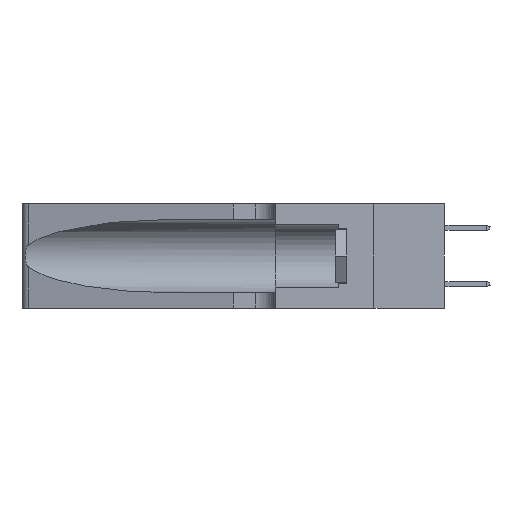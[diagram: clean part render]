
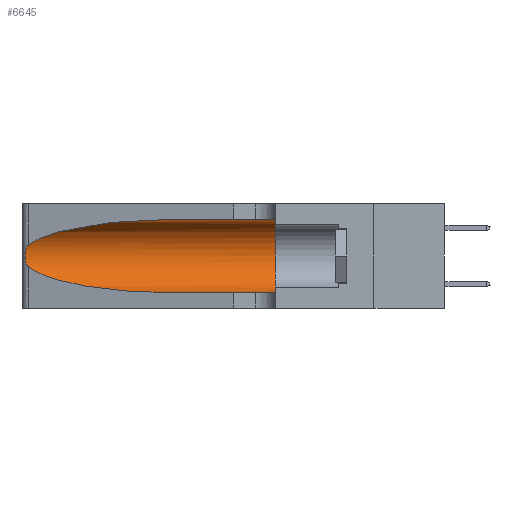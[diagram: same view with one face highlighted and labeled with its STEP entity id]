
A CAD part, left-side view. The second image highlights one B-rep face of the part: STEP entity #6645.
In plain terms, the highlighted cylindrical face has radius 3.308 mm (diameter 6.617 mm), a partial arc.
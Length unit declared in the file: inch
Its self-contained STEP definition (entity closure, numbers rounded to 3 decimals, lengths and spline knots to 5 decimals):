
#826 = VERTEX_POINT ( 'NONE', #35595 ) ;
#1830 = VECTOR ( 'NONE', #15714, 39.37008 ) ;
#2321 = DIRECTION ( 'NONE',  ( 0., -1., 0. ) ) ;
#2409 = ORIENTED_EDGE ( 'NONE', *, *, #2762, .T. ) ;
#2723 = CARTESIAN_POINT ( 'NONE',  ( 0.25487, 1.22718, 0.22369 ) ) ;
#2762 = EDGE_CURVE ( 'NONE', #18051, #28394, #26900, .T. ) ;
#2826 = EDGE_CURVE ( 'NONE', #33455, #10412, #31669, .T. ) ;
#3676 = CARTESIAN_POINT ( 'NONE',  ( 0.1305, 0.35, 0.185 ) ) ;
#4172 = CARTESIAN_POINT ( 'NONE',  ( 0.25555, 1.22994, 0.2215 ) ) ;
#4264 = B_SPLINE_CURVE_WITH_KNOTS ( 'NONE', 3,
 ( #15317, #4172, #23438, #17858, #7052, #34522, #20739, #18093, #4287, #26264, #34765, #12636, #17735, #20980 ),
 .UNSPECIFIED., .F., .F.,
 ( 4, 2, 2, 2, 2, 2, 4 ),
 ( 0., 0.00027, 0.00053, 0.00107, 0.0016, 0.00187, 0.00214 ),
 .UNSPECIFIED. ) ;
#4287 = CARTESIAN_POINT ( 'NONE',  ( 0.26017, 1.23833, 0.17102 ) ) ;
#4619 = EDGE_CURVE ( 'NONE', #826, #31121, #4264, .T. ) ;
#4683 = ORIENTED_EDGE ( 'NONE', *, *, #34054, .F. ) ;
#5385 = CARTESIAN_POINT ( 'NONE',  ( 0.1305, 0.72297, 0.31525 ) ) ;
#6645 = ADVANCED_FACE ( 'NONE', ( #24029 ), #17532, .F. ) ;
#7052 = CARTESIAN_POINT ( 'NONE',  ( 0.25854, 1.2359, 0.20912 ) ) ;
#8241 = CARTESIAN_POINT ( 'NONE',  ( 0.25487, 1.22718, 0.14631 ) ) ;
#9225 = ORIENTED_EDGE ( 'NONE', *, *, #15593, .T. ) ;
#9438 = AXIS2_PLACEMENT_3D ( 'NONE', #3676, #31109, #22939 ) ;
#10412 = VERTEX_POINT ( 'NONE', #28890 ) ;
#12636 = CARTESIAN_POINT ( 'NONE',  ( 0.25639, 1.23186, 0.15144 ) ) ;
#13640 = CARTESIAN_POINT ( 'NONE',  ( 0.18966, 0.96281, 0.31525 ) ) ;
#13798 = ORIENTED_EDGE ( 'NONE', *, *, #30500, .T. ) ;
#14192 = CARTESIAN_POINT ( 'NONE',  ( 0.1305, 0.35, 0.05475 ) ) ;
#14424 = CARTESIAN_POINT ( 'NONE',  ( 0.1305, 0.72297, 0.05475 ) ) ;
#14989 = CARTESIAN_POINT ( 'NONE',  ( 0.1305, 0.72297, 0.31525 ) ) ;
#15147 = ORIENTED_EDGE ( 'NONE', *, *, #2826, .F. ) ;
#15317 = CARTESIAN_POINT ( 'NONE',  ( 0.25487, 1.22718, 0.22369 ) ) ;
#15593 = EDGE_CURVE ( 'NONE', #31121, #18051, #31525, .T. ) ;
#15714 = DIRECTION ( 'NONE',  ( 0., -1., 0. ) ) ;
#16483 = CARTESIAN_POINT ( 'NONE',  ( 0.2373, 1.15595, 0.08982 ) ) ;
#17319 = CARTESIAN_POINT ( 'NONE',  ( 0.18966, 0.96281, 0.05475 ) ) ;
#17532 = CYLINDRICAL_SURFACE ( 'NONE', #25584, 0.13025 ) ;
#17735 = CARTESIAN_POINT ( 'NONE',  ( 0.25555, 1.22993, 0.14849 ) ) ;
#17828 = DIRECTION ( 'NONE',  ( 0., -1., 0. ) ) ;
#17858 = CARTESIAN_POINT ( 'NONE',  ( 0.25787, 1.23484, 0.2124 ) ) ;
#18051 = VERTEX_POINT ( 'NONE', #27578 ) ;
#18093 = CARTESIAN_POINT ( 'NONE',  ( 0.26075, 1.23896, 0.178 ) ) ;
#18814 = CARTESIAN_POINT ( 'NONE',  ( 0.1305, 1.61858, 0.05475 ) ) ;
#20739 = CARTESIAN_POINT ( 'NONE',  ( 0.26075, 1.23896, 0.19203 ) ) ;
#20914 = CIRCLE ( 'NONE', #9438, 0.13025 ) ;
#20980 = CARTESIAN_POINT ( 'NONE',  ( 0.25487, 1.22718, 0.14631 ) ) ;
#21201 = VECTOR ( 'NONE', #2321, 39.37008 ) ;
#21940 =( BOUNDED_CURVE ( )  B_SPLINE_CURVE ( 3, ( #5385, #13640, #27915, #2723 ),
 .UNSPECIFIED., .F., .F. ) 
 B_SPLINE_CURVE_WITH_KNOTS ( ( 4, 4 ),
 ( 1.5708, 2.84003 ),
 .UNSPECIFIED. ) 
 CURVE ( )  GEOMETRIC_REPRESENTATION_ITEM ( )  RATIONAL_B_SPLINE_CURVE ( ( 1., 0.87, 0.87, 1. ) ) 
 REPRESENTATION_ITEM ( '' )  );
#22939 = DIRECTION ( 'NONE',  ( 0., 0., 1. ) ) ;
#23408 = EDGE_LOOP ( 'NONE', ( #13798, #31059, #9225, #2409, #4683, #15147 ) ) ;
#23438 = CARTESIAN_POINT ( 'NONE',  ( 0.25639, 1.23184, 0.21858 ) ) ;
#23869 = CARTESIAN_POINT ( 'NONE',  ( 0.1305, 1.61858, 0.31525 ) ) ;
#24029 = FACE_OUTER_BOUND ( 'NONE', #23408, .T. ) ;
#25584 = AXIS2_PLACEMENT_3D ( 'NONE', #31348, #17828, #34146 ) ;
#26264 = CARTESIAN_POINT ( 'NONE',  ( 0.25856, 1.23593, 0.16098 ) ) ;
#26900 = LINE ( 'NONE', #18814, #21201 ) ;
#27578 = CARTESIAN_POINT ( 'NONE',  ( 0.1305, 0.72297, 0.05475 ) ) ;
#27915 = CARTESIAN_POINT ( 'NONE',  ( 0.2373, 1.15595, 0.28018 ) ) ;
#28394 = VERTEX_POINT ( 'NONE', #14192 ) ;
#28890 = CARTESIAN_POINT ( 'NONE',  ( 0.1305, 0.35, 0.31525 ) ) ;
#30500 = EDGE_CURVE ( 'NONE', #33455, #826, #21940, .T. ) ;
#31059 = ORIENTED_EDGE ( 'NONE', *, *, #4619, .T. ) ;
#31109 = DIRECTION ( 'NONE',  ( 0., 1., 0. ) ) ;
#31121 = VERTEX_POINT ( 'NONE', #35584 ) ;
#31348 = CARTESIAN_POINT ( 'NONE',  ( 0.1305, 1.61858, 0.185 ) ) ;
#31525 =( BOUNDED_CURVE ( )  B_SPLINE_CURVE ( 3, ( #8241, #16483, #17319, #14424 ),
 .UNSPECIFIED., .F., .F. ) 
 B_SPLINE_CURVE_WITH_KNOTS ( ( 4, 4 ),
 ( 3.44316, 4.71239 ),
 .UNSPECIFIED. ) 
 CURVE ( )  GEOMETRIC_REPRESENTATION_ITEM ( )  RATIONAL_B_SPLINE_CURVE ( ( 1., 0.87, 0.87, 1. ) ) 
 REPRESENTATION_ITEM ( '' )  );
#31669 = LINE ( 'NONE', #23869, #1830 ) ;
#33455 = VERTEX_POINT ( 'NONE', #14989 ) ;
#34054 = EDGE_CURVE ( 'NONE', #10412, #28394, #20914, .T. ) ;
#34146 = DIRECTION ( 'NONE',  ( 0., 0., -1. ) ) ;
#34522 = CARTESIAN_POINT ( 'NONE',  ( 0.26018, 1.23835, 0.19895 ) ) ;
#34765 = CARTESIAN_POINT ( 'NONE',  ( 0.25789, 1.23486, 0.15765 ) ) ;
#35584 = CARTESIAN_POINT ( 'NONE',  ( 0.25487, 1.22718, 0.14631 ) ) ;
#35595 = CARTESIAN_POINT ( 'NONE',  ( 0.25487, 1.22718, 0.22369 ) ) ;
